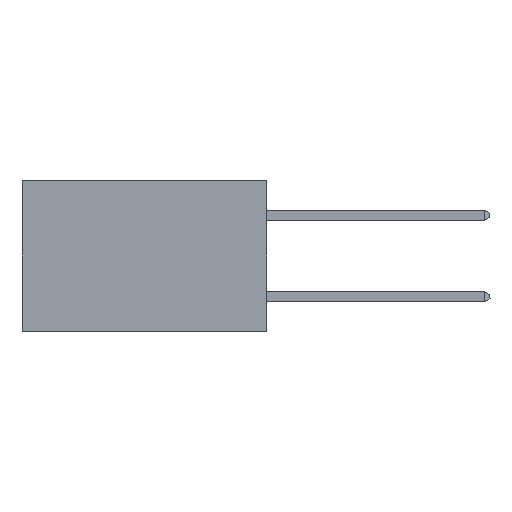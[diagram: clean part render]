
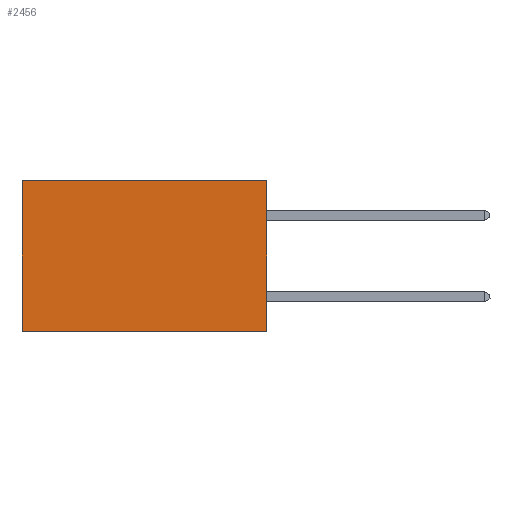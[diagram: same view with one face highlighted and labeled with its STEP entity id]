
A CAD part, left-side view. The second image highlights one B-rep face of the part: STEP entity #2456.
In plain terms, the highlighted planar face has unit normal (-1, 0, 0).
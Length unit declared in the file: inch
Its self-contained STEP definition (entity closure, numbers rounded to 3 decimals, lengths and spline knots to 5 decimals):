
#153 = FACE_OUTER_BOUND ( 'NONE', #848, .T. ) ;
#186 = DIRECTION ( 'NONE',  ( 0., 1., 0. ) ) ;
#371 = VERTEX_POINT ( 'NONE', #9207 ) ;
#848 = EDGE_LOOP ( 'NONE', ( #9180, #8081, #7839, #1877 ) ) ;
#965 = EDGE_CURVE ( 'NONE', #9545, #371, #5332, .T. ) ;
#1149 = DIRECTION ( 'NONE',  ( 1., 0., 0. ) ) ;
#1284 = VECTOR ( 'NONE', #3863, 39.37008 ) ;
#1664 = EDGE_CURVE ( 'NONE', #8780, #2768, #9176, .T. ) ;
#1829 = CARTESIAN_POINT ( 'NONE',  ( 0.2875, 0.6, 0. ) ) ;
#1873 = VECTOR ( 'NONE', #9411, 39.37008 ) ;
#1877 = ORIENTED_EDGE ( 'NONE', *, *, #3240, .T. ) ;
#2407 = VECTOR ( 'NONE', #186, 39.37008 ) ;
#2456 = ADVANCED_FACE ( 'NONE', ( #153 ), #3440, .F. ) ;
#2601 = CARTESIAN_POINT ( 'NONE',  ( 0.2875, 0.6, 0. ) ) ;
#2624 = AXIS2_PLACEMENT_3D ( 'NONE', #9592, #1149, #5671 ) ;
#2718 = DIRECTION ( 'NONE',  ( 0., 1., 0. ) ) ;
#2768 = VERTEX_POINT ( 'NONE', #4124 ) ;
#3240 = EDGE_CURVE ( 'NONE', #9545, #8780, #5398, .T. ) ;
#3440 = PLANE ( 'NONE',  #2624 ) ;
#3863 = DIRECTION ( 'NONE',  ( 0., 0., -1. ) ) ;
#4092 = EDGE_CURVE ( 'NONE', #371, #2768, #4523, .T. ) ;
#4124 = CARTESIAN_POINT ( 'NONE',  ( 0.2875, 0.6, -0.37 ) ) ;
#4523 = LINE ( 'NONE', #7291, #5752 ) ;
#4895 = CARTESIAN_POINT ( 'NONE',  ( 0.2875, 0., 0. ) ) ;
#5332 = LINE ( 'NONE', #7709, #1284 ) ;
#5398 = LINE ( 'NONE', #6343, #2407 ) ;
#5671 = DIRECTION ( 'NONE',  ( 0., 0., -1. ) ) ;
#5752 = VECTOR ( 'NONE', #2718, 39.37008 ) ;
#6343 = CARTESIAN_POINT ( 'NONE',  ( 0.2875, 0., 0. ) ) ;
#7291 = CARTESIAN_POINT ( 'NONE',  ( 0.2875, 0., -0.37 ) ) ;
#7709 = CARTESIAN_POINT ( 'NONE',  ( 0.2875, 0., 0. ) ) ;
#7839 = ORIENTED_EDGE ( 'NONE', *, *, #965, .F. ) ;
#8081 = ORIENTED_EDGE ( 'NONE', *, *, #4092, .F. ) ;
#8780 = VERTEX_POINT ( 'NONE', #2601 ) ;
#9176 = LINE ( 'NONE', #1829, #1873 ) ;
#9180 = ORIENTED_EDGE ( 'NONE', *, *, #1664, .T. ) ;
#9207 = CARTESIAN_POINT ( 'NONE',  ( 0.2875, 0., -0.37 ) ) ;
#9411 = DIRECTION ( 'NONE',  ( 0., 0., -1. ) ) ;
#9545 = VERTEX_POINT ( 'NONE', #4895 ) ;
#9592 = CARTESIAN_POINT ( 'NONE',  ( 0.2875, 0., 0. ) ) ;
